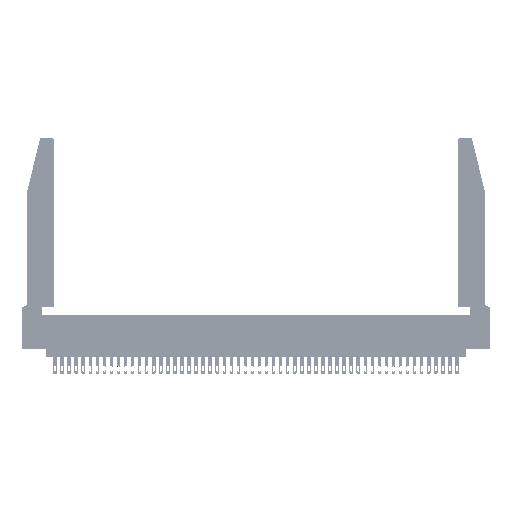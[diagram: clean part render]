
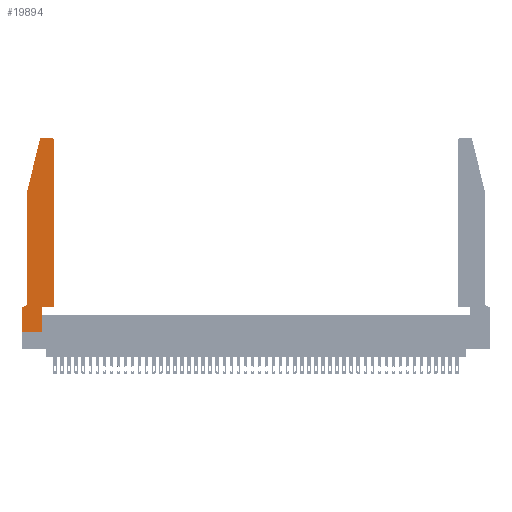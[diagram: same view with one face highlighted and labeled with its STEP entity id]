
A CAD part, top view. The second image highlights one B-rep face of the part: STEP entity #19894.
In plain terms, the highlighted planar face has unit normal (0, 0, 1).
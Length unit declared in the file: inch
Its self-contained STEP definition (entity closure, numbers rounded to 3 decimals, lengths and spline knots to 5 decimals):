
#102 = CARTESIAN_POINT ( 'NONE',  ( 0.4505, 0.35, 0.37 ) ) ;
#490 = DIRECTION ( 'NONE',  ( 0., 1., 0. ) ) ;
#554 = VECTOR ( 'NONE', #31686, 39.37008 ) ;
#709 = VERTEX_POINT ( 'NONE', #2125 ) ;
#1700 = ORIENTED_EDGE ( 'NONE', *, *, #17187, .T. ) ;
#2125 = CARTESIAN_POINT ( 'NONE',  ( 0.4205, 2.75, 0.37 ) ) ;
#2321 = DIRECTION ( 'NONE',  ( 0., 0., 1. ) ) ;
#2371 = VERTEX_POINT ( 'NONE', #17292 ) ;
#2534 = EDGE_CURVE ( 'NONE', #47191, #7977, #4205, .T. ) ;
#2821 = ORIENTED_EDGE ( 'NONE', *, *, #28475, .T. ) ;
#3912 = CARTESIAN_POINT ( 'NONE',  ( 0.4505, 0.35, 0.37 ) ) ;
#3986 = VERTEX_POINT ( 'NONE', #44077 ) ;
#4150 = VECTOR ( 'NONE', #41358, 39.37008 ) ;
#4205 = LINE ( 'NONE', #30441, #42598 ) ;
#4741 = VECTOR ( 'NONE', #44982, 39.37008 ) ;
#5371 = PLANE ( 'NONE',  #30054 ) ;
#6758 = CIRCLE ( 'NONE', #23990, 0.07 ) ;
#7559 = EDGE_CURVE ( 'NONE', #24186, #16036, #6758, .T. ) ;
#7977 = VERTEX_POINT ( 'NONE', #23484 ) ;
#8055 = ORIENTED_EDGE ( 'NONE', *, *, #22907, .T. ) ;
#9394 = DIRECTION ( 'NONE',  ( 0., -1., 0. ) ) ;
#9406 = CARTESIAN_POINT ( 'NONE',  ( 0.0055, 0.42, 0.37 ) ) ;
#9886 = CARTESIAN_POINT ( 'NONE',  ( 0.284, 2.72, 0.37 ) ) ;
#10281 = EDGE_CURVE ( 'NONE', #10619, #19558, #16373, .T. ) ;
#10599 = VERTEX_POINT ( 'NONE', #102 ) ;
#10619 = VERTEX_POINT ( 'NONE', #40881 ) ;
#12629 = LINE ( 'NONE', #16665, #41710 ) ;
#12823 = LINE ( 'NONE', #3912, #34908 ) ;
#12871 = DIRECTION ( 'NONE',  ( 1., 0., 0. ) ) ;
#13446 = DIRECTION ( 'NONE',  ( 0., 0., 1. ) ) ;
#13540 = CARTESIAN_POINT ( 'NONE',  ( 0., 0.35, 0.37 ) ) ;
#13724 = DIRECTION ( 'NONE',  ( 1., 0., 0. ) ) ;
#14953 = CARTESIAN_POINT ( 'NONE',  ( 0.25487, 2.72718, 0.37 ) ) ;
#16036 = VERTEX_POINT ( 'NONE', #31903 ) ;
#16373 = CIRCLE ( 'NONE', #42732, 0.03 ) ;
#16665 = CARTESIAN_POINT ( 'NONE',  ( 0., 0., 0.37 ) ) ;
#17187 = EDGE_CURVE ( 'NONE', #2371, #24186, #19008, .T. ) ;
#17292 = CARTESIAN_POINT ( 'NONE',  ( 0.0755, 2., 0.37 ) ) ;
#17715 = VERTEX_POINT ( 'NONE', #24913 ) ;
#18825 = DIRECTION ( 'NONE',  ( -0.239, -0.971, 0. ) ) ;
#19008 = LINE ( 'NONE', #31640, #43441 ) ;
#19147 = ORIENTED_EDGE ( 'NONE', *, *, #28925, .T. ) ;
#19558 = VERTEX_POINT ( 'NONE', #14953 ) ;
#19894 = ADVANCED_FACE ( 'NONE', ( #33391 ), #5371, .T. ) ;
#20255 = CARTESIAN_POINT ( 'NONE',  ( 0.4505, 0.35, 0.37 ) ) ;
#20896 = CARTESIAN_POINT ( 'NONE',  ( 0.2865, 0., 0.37 ) ) ;
#21409 = VERTEX_POINT ( 'NONE', #13540 ) ;
#21539 = ORIENTED_EDGE ( 'NONE', *, *, #42183, .T. ) ;
#22200 = ORIENTED_EDGE ( 'NONE', *, *, #2534, .T. ) ;
#22907 = EDGE_CURVE ( 'NONE', #16036, #21409, #24524, .T. ) ;
#23484 = CARTESIAN_POINT ( 'NONE',  ( 0.2865, 0.35, 0.37 ) ) ;
#23987 = DIRECTION ( 'NONE',  ( 1., 0., 0. ) ) ;
#23990 = AXIS2_PLACEMENT_3D ( 'NONE', #9406, #28392, #46952 ) ;
#24186 = VERTEX_POINT ( 'NONE', #42462 ) ;
#24524 = LINE ( 'NONE', #37623, #4741 ) ;
#24913 = CARTESIAN_POINT ( 'NONE',  ( 0.4505, 2.72, 0.37 ) ) ;
#26710 = LINE ( 'NONE', #38985, #554 ) ;
#27434 = LINE ( 'NONE', #41045, #4150 ) ;
#27763 = ORIENTED_EDGE ( 'NONE', *, *, #38660, .T. ) ;
#28392 = DIRECTION ( 'NONE',  ( 0., 0., -1. ) ) ;
#28475 = EDGE_CURVE ( 'NONE', #709, #10619, #26710, .T. ) ;
#28925 = EDGE_CURVE ( 'NONE', #7977, #10599, #38979, .T. ) ;
#28955 = ORIENTED_EDGE ( 'NONE', *, *, #44470, .T. ) ;
#29833 = CARTESIAN_POINT ( 'NONE',  ( 0.0755, 2., 0.37 ) ) ;
#29988 = ORIENTED_EDGE ( 'NONE', *, *, #10281, .T. ) ;
#30054 = AXIS2_PLACEMENT_3D ( 'NONE', #38849, #35125, #12871 ) ;
#30057 = EDGE_CURVE ( 'NONE', #10599, #17715, #12823, .T. ) ;
#30441 = CARTESIAN_POINT ( 'NONE',  ( 0.2865, 0.35, 0.37 ) ) ;
#31158 = CIRCLE ( 'NONE', #46958, 0.03 ) ;
#31426 = DIRECTION ( 'NONE',  ( 0., -1., 0. ) ) ;
#31640 = CARTESIAN_POINT ( 'NONE',  ( 0.0755, 2., 0.37 ) ) ;
#31686 = DIRECTION ( 'NONE',  ( -1., 0., 0. ) ) ;
#31903 = CARTESIAN_POINT ( 'NONE',  ( 0.0055, 0.35, 0.37 ) ) ;
#31904 = CARTESIAN_POINT ( 'NONE',  ( 0.4205, 2.72, 0.37 ) ) ;
#31976 = VECTOR ( 'NONE', #23987, 39.37008 ) ;
#32658 = EDGE_LOOP ( 'NONE', ( #2821, #29988, #43097, #1700, #34775, #8055, #28955, #27763, #22200, #19147, #47256, #21539 ) ) ;
#33391 = FACE_OUTER_BOUND ( 'NONE', #32658, .T. ) ;
#34775 = ORIENTED_EDGE ( 'NONE', *, *, #7559, .T. ) ;
#34908 = VECTOR ( 'NONE', #490, 39.37008 ) ;
#35125 = DIRECTION ( 'NONE',  ( 0., 0., 1. ) ) ;
#36083 = VECTOR ( 'NONE', #18825, 39.37008 ) ;
#37623 = CARTESIAN_POINT ( 'NONE',  ( 0.0755, 0.35, 0.37 ) ) ;
#38660 = EDGE_CURVE ( 'NONE', #3986, #47191, #27434, .T. ) ;
#38684 = EDGE_CURVE ( 'NONE', #19558, #2371, #39625, .T. ) ;
#38849 = CARTESIAN_POINT ( 'NONE',  ( 0., 0.35, 0.37 ) ) ;
#38979 = LINE ( 'NONE', #20255, #31976 ) ;
#38985 = CARTESIAN_POINT ( 'NONE',  ( 0.2605, 2.75, 0.37 ) ) ;
#39421 = DIRECTION ( 'NONE',  ( 1., 0., 0. ) ) ;
#39625 = LINE ( 'NONE', #29833, #36083 ) ;
#40881 = CARTESIAN_POINT ( 'NONE',  ( 0.284, 2.75, 0.37 ) ) ;
#41045 = CARTESIAN_POINT ( 'NONE',  ( 0., 0., 0.37 ) ) ;
#41358 = DIRECTION ( 'NONE',  ( 1., 0., 0. ) ) ;
#41710 = VECTOR ( 'NONE', #31426, 39.37008 ) ;
#42183 = EDGE_CURVE ( 'NONE', #17715, #709, #31158, .T. ) ;
#42462 = CARTESIAN_POINT ( 'NONE',  ( 0.0755, 0.42, 0.37 ) ) ;
#42598 = VECTOR ( 'NONE', #47975, 39.37008 ) ;
#42732 = AXIS2_PLACEMENT_3D ( 'NONE', #9886, #13446, #39421 ) ;
#43097 = ORIENTED_EDGE ( 'NONE', *, *, #38684, .T. ) ;
#43441 = VECTOR ( 'NONE', #9394, 39.37008 ) ;
#44077 = CARTESIAN_POINT ( 'NONE',  ( 0., 0., 0.37 ) ) ;
#44470 = EDGE_CURVE ( 'NONE', #21409, #3986, #12629, .T. ) ;
#44982 = DIRECTION ( 'NONE',  ( -1., 0., 0. ) ) ;
#46952 = DIRECTION ( 'NONE',  ( -1., 0., 0. ) ) ;
#46958 = AXIS2_PLACEMENT_3D ( 'NONE', #31904, #2321, #13724 ) ;
#47191 = VERTEX_POINT ( 'NONE', #20896 ) ;
#47256 = ORIENTED_EDGE ( 'NONE', *, *, #30057, .T. ) ;
#47975 = DIRECTION ( 'NONE',  ( 0., 1., 0. ) ) ;
